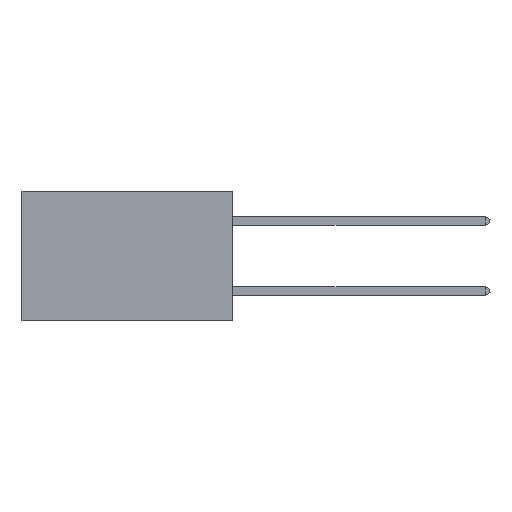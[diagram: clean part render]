
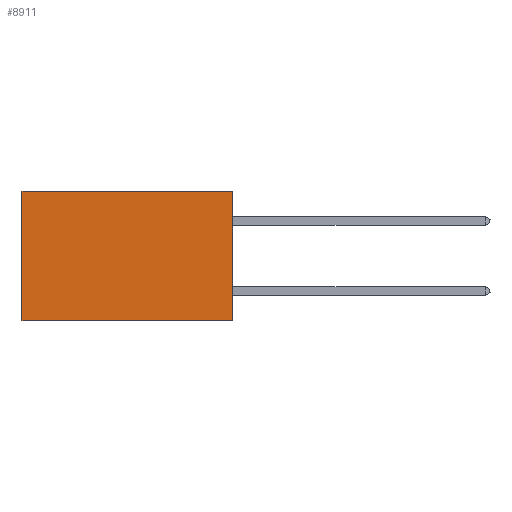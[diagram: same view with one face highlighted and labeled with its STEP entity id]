
A CAD part, left-side view. The second image highlights one B-rep face of the part: STEP entity #8911.
In plain terms, the highlighted face is planar.
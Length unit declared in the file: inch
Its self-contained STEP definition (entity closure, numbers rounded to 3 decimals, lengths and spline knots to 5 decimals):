
#182 = VECTOR ( 'NONE', #17205, 39.37008 ) ;
#2035 = DIRECTION ( 'NONE',  ( 0., 1., 0. ) ) ;
#2787 = AXIS2_PLACEMENT_3D ( 'NONE', #16270, #8871, #13018 ) ;
#4105 = CARTESIAN_POINT ( 'NONE',  ( 0.2875, 0., 0. ) ) ;
#6836 = CARTESIAN_POINT ( 'NONE',  ( 0.2875, 0., -0.37 ) ) ;
#8871 = DIRECTION ( 'NONE',  ( 1., 0., 0. ) ) ;
#8911 = ADVANCED_FACE ( 'NONE', ( #17228 ), #40124, .F. ) ;
#9927 = LINE ( 'NONE', #33203, #10581 ) ;
#10581 = VECTOR ( 'NONE', #2035, 39.37008 ) ;
#10830 = ORIENTED_EDGE ( 'NONE', *, *, #25323, .F. ) ;
#13018 = DIRECTION ( 'NONE',  ( 0., 0., -1. ) ) ;
#14724 = ORIENTED_EDGE ( 'NONE', *, *, #29935, .T. ) ;
#16018 = VECTOR ( 'NONE', #43238, 39.37008 ) ;
#16270 = CARTESIAN_POINT ( 'NONE',  ( 0.2875, 0., 0. ) ) ;
#16800 = VECTOR ( 'NONE', #50092, 39.37008 ) ;
#17205 = DIRECTION ( 'NONE',  ( 0., 1., 0. ) ) ;
#17228 = FACE_OUTER_BOUND ( 'NONE', #31118, .T. ) ;
#18897 = CARTESIAN_POINT ( 'NONE',  ( 0.2875, 0.6, 0. ) ) ;
#21076 = LINE ( 'NONE', #18897, #16800 ) ;
#23559 = ORIENTED_EDGE ( 'NONE', *, *, #38250, .F. ) ;
#24717 = VERTEX_POINT ( 'NONE', #44917 ) ;
#24727 = CARTESIAN_POINT ( 'NONE',  ( 0.2875, 0.6, -0.37 ) ) ;
#25323 = EDGE_CURVE ( 'NONE', #26718, #40348, #9927, .T. ) ;
#26440 = LINE ( 'NONE', #38980, #16018 ) ;
#26718 = VERTEX_POINT ( 'NONE', #6836 ) ;
#29935 = EDGE_CURVE ( 'NONE', #24717, #40348, #21076, .T. ) ;
#31118 = EDGE_LOOP ( 'NONE', ( #14724, #10830, #23559, #42780 ) ) ;
#31635 = EDGE_CURVE ( 'NONE', #32666, #24717, #34477, .T. ) ;
#32666 = VERTEX_POINT ( 'NONE', #4105 ) ;
#33203 = CARTESIAN_POINT ( 'NONE',  ( 0.2875, 0., -0.37 ) ) ;
#34477 = LINE ( 'NONE', #40713, #182 ) ;
#38250 = EDGE_CURVE ( 'NONE', #32666, #26718, #26440, .T. ) ;
#38980 = CARTESIAN_POINT ( 'NONE',  ( 0.2875, 0., 0. ) ) ;
#40124 = PLANE ( 'NONE',  #2787 ) ;
#40348 = VERTEX_POINT ( 'NONE', #24727 ) ;
#40713 = CARTESIAN_POINT ( 'NONE',  ( 0.2875, 0., 0. ) ) ;
#42780 = ORIENTED_EDGE ( 'NONE', *, *, #31635, .T. ) ;
#43238 = DIRECTION ( 'NONE',  ( 0., 0., -1. ) ) ;
#44917 = CARTESIAN_POINT ( 'NONE',  ( 0.2875, 0.6, 0. ) ) ;
#50092 = DIRECTION ( 'NONE',  ( 0., 0., -1. ) ) ;
